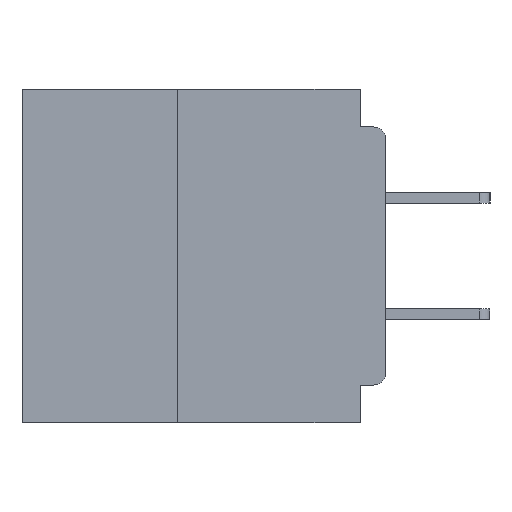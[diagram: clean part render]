
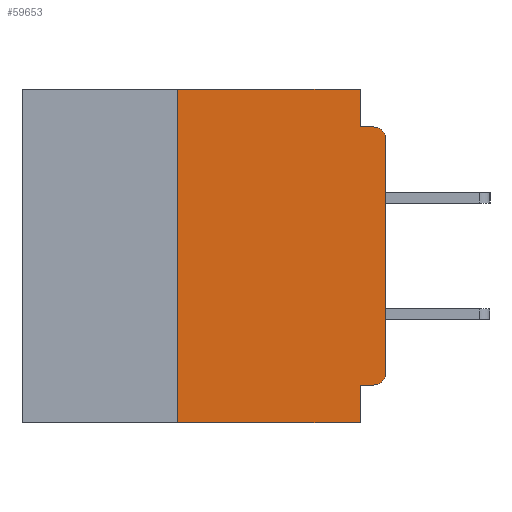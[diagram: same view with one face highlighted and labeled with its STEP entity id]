
A CAD part, left-side view. The second image highlights one B-rep face of the part: STEP entity #59653.
In plain terms, the highlighted planar face has unit normal (-1, 0, 0).
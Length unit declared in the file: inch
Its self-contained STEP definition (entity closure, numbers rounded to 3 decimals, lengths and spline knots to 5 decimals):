
#1578 = AXIS2_PLACEMENT_3D ( 'NONE', #32272, #17895, #51687 ) ;
#4415 = VERTEX_POINT ( 'NONE', #62027 ) ;
#5528 = CARTESIAN_POINT ( 'NONE',  ( 0., 0., -0.34 ) ) ;
#8045 = ORIENTED_EDGE ( 'NONE', *, *, #61714, .T. ) ;
#8489 = CIRCLE ( 'NONE', #39140, 0.015 ) ;
#9659 = CARTESIAN_POINT ( 'NONE',  ( 0., 0., 0. ) ) ;
#9825 = ORIENTED_EDGE ( 'NONE', *, *, #57488, .T. ) ;
#10280 = CIRCLE ( 'NONE', #49507, 0.015 ) ;
#11060 = VERTEX_POINT ( 'NONE', #33049 ) ;
#11209 = VECTOR ( 'NONE', #48423, 39.37008 ) ;
#12487 = VECTOR ( 'NONE', #45781, 39.37008 ) ;
#12861 = CARTESIAN_POINT ( 'NONE',  ( 0., 0.031, 0. ) ) ;
#13040 = PLANE ( 'NONE',  #1578 ) ;
#15147 = DIRECTION ( 'NONE',  ( -1., 0., 0. ) ) ;
#15185 = EDGE_CURVE ( 'NONE', #39696, #4415, #31391, .T. ) ;
#16232 = ORIENTED_EDGE ( 'NONE', *, *, #60082, .F. ) ;
#16620 = DIRECTION ( 'NONE',  ( 0., 1., 0. ) ) ;
#17236 = ORIENTED_EDGE ( 'NONE', *, *, #15185, .F. ) ;
#17602 = LINE ( 'NONE', #50994, #54654 ) ;
#17895 = DIRECTION ( 'NONE',  ( 1., 0., 0. ) ) ;
#18532 = VECTOR ( 'NONE', #27597, 39.37008 ) ;
#19383 = DIRECTION ( 'NONE',  ( 0., 0., 1. ) ) ;
#21974 = DIRECTION ( 'NONE',  ( -1., 0., 0. ) ) ;
#22080 = DIRECTION ( 'NONE',  ( 0., 0., -1. ) ) ;
#23239 = EDGE_CURVE ( 'NONE', #58201, #32223, #8489, .T. ) ;
#24188 = CARTESIAN_POINT ( 'NONE',  ( 0., 0.437, 0. ) ) ;
#26368 = CARTESIAN_POINT ( 'NONE',  ( 0., 0., -0.045 ) ) ;
#26678 = EDGE_LOOP ( 'NONE', ( #48017, #8045, #41606, #37667, #56139, #17236, #9825, #16232, #35848, #46367 ) ) ;
#27474 = CARTESIAN_POINT ( 'NONE',  ( 0., 0.031, -0.4 ) ) ;
#27597 = DIRECTION ( 'NONE',  ( 0., 0., 1. ) ) ;
#27740 = VERTEX_POINT ( 'NONE', #27474 ) ;
#28015 = CARTESIAN_POINT ( 'NONE',  ( 0., 0.031, -0.355 ) ) ;
#28409 = VECTOR ( 'NONE', #16620, 39.37008 ) ;
#29896 = CARTESIAN_POINT ( 'NONE',  ( 0., 0.25, -0.4 ) ) ;
#30023 = CARTESIAN_POINT ( 'NONE',  ( 0., 0.031, -0.045 ) ) ;
#31391 = LINE ( 'NONE', #51639, #18532 ) ;
#32073 = DIRECTION ( 'NONE',  ( 0., -1., 0. ) ) ;
#32223 = VERTEX_POINT ( 'NONE', #5528 ) ;
#32272 = CARTESIAN_POINT ( 'NONE',  ( 0., 0.437, 0. ) ) ;
#33049 = CARTESIAN_POINT ( 'NONE',  ( 0., 0.015, -0.045 ) ) ;
#35385 = EDGE_CURVE ( 'NONE', #4415, #45389, #48222, .T. ) ;
#35848 = ORIENTED_EDGE ( 'NONE', *, *, #37057, .F. ) ;
#36662 = DIRECTION ( 'NONE',  ( 0., 0., -1. ) ) ;
#36937 = CARTESIAN_POINT ( 'NONE',  ( 0., 0.437, -0.4 ) ) ;
#37057 = EDGE_CURVE ( 'NONE', #58201, #53123, #54081, .T. ) ;
#37131 = EDGE_CURVE ( 'NONE', #38582, #11060, #51015, .T. ) ;
#37667 = ORIENTED_EDGE ( 'NONE', *, *, #47755, .F. ) ;
#38582 = VERTEX_POINT ( 'NONE', #30023 ) ;
#39140 = AXIS2_PLACEMENT_3D ( 'NONE', #50890, #21974, #55777 ) ;
#39696 = VERTEX_POINT ( 'NONE', #29896 ) ;
#40051 = VERTEX_POINT ( 'NONE', #42279 ) ;
#41606 = ORIENTED_EDGE ( 'NONE', *, *, #37131, .F. ) ;
#41813 = VECTOR ( 'NONE', #32073, 39.37008 ) ;
#42279 = CARTESIAN_POINT ( 'NONE',  ( 0., 0., -0.06 ) ) ;
#43808 = EDGE_CURVE ( 'NONE', #32223, #40051, #58865, .T. ) ;
#44060 = CARTESIAN_POINT ( 'NONE',  ( 0., 0.015, -0.06 ) ) ;
#45389 = VERTEX_POINT ( 'NONE', #12861 ) ;
#45781 = DIRECTION ( 'NONE',  ( 0., -1., 0. ) ) ;
#46010 = VECTOR ( 'NONE', #19383, 39.37008 ) ;
#46162 = CARTESIAN_POINT ( 'NONE',  ( 0., 0.031, -0.4 ) ) ;
#46367 = ORIENTED_EDGE ( 'NONE', *, *, #23239, .T. ) ;
#47755 = EDGE_CURVE ( 'NONE', #45389, #38582, #17602, .T. ) ;
#48017 = ORIENTED_EDGE ( 'NONE', *, *, #43808, .T. ) ;
#48222 = LINE ( 'NONE', #24188, #11209 ) ;
#48423 = DIRECTION ( 'NONE',  ( 0., -1., 0. ) ) ;
#48919 = DIRECTION ( 'NONE',  ( 0., 0., -1. ) ) ;
#49507 = AXIS2_PLACEMENT_3D ( 'NONE', #44060, #15147, #48919 ) ;
#50200 = CARTESIAN_POINT ( 'NONE',  ( 0., 0., -0.355 ) ) ;
#50890 = CARTESIAN_POINT ( 'NONE',  ( 0., 0.015, -0.34 ) ) ;
#50994 = CARTESIAN_POINT ( 'NONE',  ( 0., 0.031, 0. ) ) ;
#51015 = LINE ( 'NONE', #26368, #12487 ) ;
#51275 = LINE ( 'NONE', #46162, #62582 ) ;
#51639 = CARTESIAN_POINT ( 'NONE',  ( 0., 0.25, -0.4 ) ) ;
#51687 = DIRECTION ( 'NONE',  ( 0., 0., -1. ) ) ;
#52033 = CARTESIAN_POINT ( 'NONE',  ( 0., 0.015, -0.355 ) ) ;
#52880 = FACE_OUTER_BOUND ( 'NONE', #26678, .T. ) ;
#53123 = VERTEX_POINT ( 'NONE', #28015 ) ;
#54081 = LINE ( 'NONE', #50200, #28409 ) ;
#54654 = VECTOR ( 'NONE', #36662, 39.37008 ) ;
#55777 = DIRECTION ( 'NONE',  ( 0., 0., -1. ) ) ;
#56139 = ORIENTED_EDGE ( 'NONE', *, *, #35385, .F. ) ;
#56199 = LINE ( 'NONE', #36937, #41813 ) ;
#57488 = EDGE_CURVE ( 'NONE', #39696, #27740, #56199, .T. ) ;
#58201 = VERTEX_POINT ( 'NONE', #52033 ) ;
#58865 = LINE ( 'NONE', #9659, #46010 ) ;
#59653 = ADVANCED_FACE ( 'NONE', ( #52880 ), #13040, .F. ) ;
#60082 = EDGE_CURVE ( 'NONE', #53123, #27740, #51275, .T. ) ;
#61714 = EDGE_CURVE ( 'NONE', #40051, #11060, #10280, .T. ) ;
#62027 = CARTESIAN_POINT ( 'NONE',  ( 0., 0.25, 0. ) ) ;
#62582 = VECTOR ( 'NONE', #22080, 39.37008 ) ;
